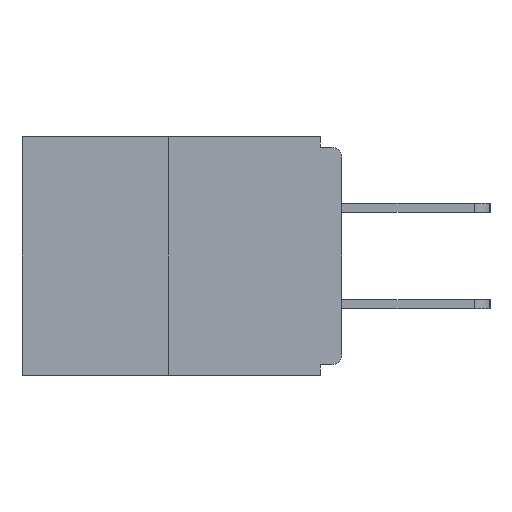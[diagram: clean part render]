
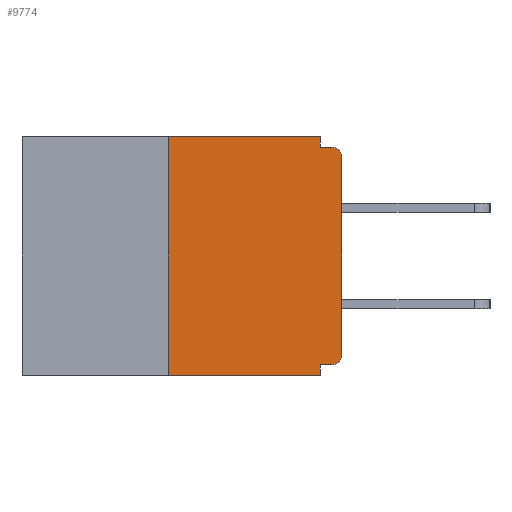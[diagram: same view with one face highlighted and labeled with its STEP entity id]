
A CAD part, left-side view. The second image highlights one B-rep face of the part: STEP entity #9774.
In plain terms, the highlighted planar face has unit normal (-1, 0, 0).
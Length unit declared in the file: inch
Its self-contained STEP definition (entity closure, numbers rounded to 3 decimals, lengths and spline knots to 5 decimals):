
#645 = ORIENTED_EDGE ( 'NONE', *, *, #3847, .F. ) ;
#1141 = VECTOR ( 'NONE', #11900, 39.37008 ) ;
#1567 = EDGE_CURVE ( 'NONE', #14206, #4129, #3228, .T. ) ;
#2393 = LINE ( 'NONE', #6548, #3280 ) ;
#2454 = DIRECTION ( 'NONE',  ( 0., -1., 0. ) ) ;
#2554 = AXIS2_PLACEMENT_3D ( 'NONE', #10308, #8791, #17284 ) ;
#2558 = DIRECTION ( 'NONE',  ( 0., 0., 1. ) ) ;
#2584 = VERTEX_POINT ( 'NONE', #14628 ) ;
#2703 = VERTEX_POINT ( 'NONE', #7894 ) ;
#2985 = CARTESIAN_POINT ( 'NONE',  ( 0., 0.031, -0.328 ) ) ;
#3004 = DIRECTION ( 'NONE',  ( -1., 0., 0. ) ) ;
#3228 = CIRCLE ( 'NONE', #16253, 0.015 ) ;
#3280 = VECTOR ( 'NONE', #12110, 39.37008 ) ;
#3322 = PLANE ( 'NONE',  #2554 ) ;
#3410 = EDGE_CURVE ( 'NONE', #3979, #9281, #3628, .T. ) ;
#3470 = VECTOR ( 'NONE', #2454, 39.37008 ) ;
#3628 = LINE ( 'NONE', #5247, #3470 ) ;
#3847 = EDGE_CURVE ( 'NONE', #2703, #13763, #7353, .T. ) ;
#3947 = VECTOR ( 'NONE', #14082, 39.37008 ) ;
#3979 = VERTEX_POINT ( 'NONE', #7965 ) ;
#4129 = VERTEX_POINT ( 'NONE', #14866 ) ;
#4178 = CARTESIAN_POINT ( 'NONE',  ( 0., 0.015, -0.313 ) ) ;
#4194 = CARTESIAN_POINT ( 'NONE',  ( 0., 0.031, -0.343 ) ) ;
#4447 = DIRECTION ( 'NONE',  ( 0., 0., -1. ) ) ;
#4765 = FACE_OUTER_BOUND ( 'NONE', #6492, .T. ) ;
#5152 = ORIENTED_EDGE ( 'NONE', *, *, #13144, .F. ) ;
#5247 = CARTESIAN_POINT ( 'NONE',  ( 0., 0.46, -0.343 ) ) ;
#5688 = VECTOR ( 'NONE', #2558, 39.37008 ) ;
#5860 = VECTOR ( 'NONE', #14161, 39.37008 ) ;
#6120 = LINE ( 'NONE', #17193, #14213 ) ;
#6492 = EDGE_LOOP ( 'NONE', ( #17473, #10334, #14534, #16892, #6606, #6872, #6657, #11064, #5152, #645 ) ) ;
#6548 = CARTESIAN_POINT ( 'NONE',  ( 0., 0.46, 0. ) ) ;
#6606 = ORIENTED_EDGE ( 'NONE', *, *, #14551, .F. ) ;
#6657 = ORIENTED_EDGE ( 'NONE', *, *, #17885, .T. ) ;
#6781 = EDGE_CURVE ( 'NONE', #9691, #9281, #13333, .T. ) ;
#6872 = ORIENTED_EDGE ( 'NONE', *, *, #1567, .T. ) ;
#6930 = AXIS2_PLACEMENT_3D ( 'NONE', #12238, #14766, #17742 ) ;
#7265 = CARTESIAN_POINT ( 'NONE',  ( 0., 0., -0.328 ) ) ;
#7353 = LINE ( 'NONE', #8737, #3947 ) ;
#7894 = CARTESIAN_POINT ( 'NONE',  ( 0., 0.031, 0. ) ) ;
#7965 = CARTESIAN_POINT ( 'NONE',  ( 0., 0.25, -0.343 ) ) ;
#8478 = VERTEX_POINT ( 'NONE', #16604 ) ;
#8737 = CARTESIAN_POINT ( 'NONE',  ( 0., 0.031, 0. ) ) ;
#8791 = DIRECTION ( 'NONE',  ( 1., 0., 0. ) ) ;
#9272 = EDGE_CURVE ( 'NONE', #3979, #2584, #14990, .T. ) ;
#9281 = VERTEX_POINT ( 'NONE', #4194 ) ;
#9298 = VECTOR ( 'NONE', #4447, 39.37008 ) ;
#9691 = VERTEX_POINT ( 'NONE', #2985 ) ;
#9716 = DIRECTION ( 'NONE',  ( 0., 0., -1. ) ) ;
#9774 = ADVANCED_FACE ( 'NONE', ( #4765 ), #3322, .F. ) ;
#10272 = CARTESIAN_POINT ( 'NONE',  ( 0., 0.015, -0.328 ) ) ;
#10308 = CARTESIAN_POINT ( 'NONE',  ( 0., 0.46, 0. ) ) ;
#10334 = ORIENTED_EDGE ( 'NONE', *, *, #9272, .F. ) ;
#11064 = ORIENTED_EDGE ( 'NONE', *, *, #17128, .T. ) ;
#11674 = CARTESIAN_POINT ( 'NONE',  ( 0., 0.031, -0.015 ) ) ;
#11900 = DIRECTION ( 'NONE',  ( 0., 0., 1. ) ) ;
#12110 = DIRECTION ( 'NONE',  ( 0., -1., 0. ) ) ;
#12238 = CARTESIAN_POINT ( 'NONE',  ( 0., 0.015, -0.03 ) ) ;
#12731 = VERTEX_POINT ( 'NONE', #16027 ) ;
#13144 = EDGE_CURVE ( 'NONE', #13763, #12731, #6120, .T. ) ;
#13333 = LINE ( 'NONE', #14588, #9298 ) ;
#13763 = VERTEX_POINT ( 'NONE', #11674 ) ;
#14082 = DIRECTION ( 'NONE',  ( 0., 0., -1. ) ) ;
#14161 = DIRECTION ( 'NONE',  ( 0., 1., 0. ) ) ;
#14179 = CIRCLE ( 'NONE', #6930, 0.015 ) ;
#14206 = VERTEX_POINT ( 'NONE', #10272 ) ;
#14213 = VECTOR ( 'NONE', #15926, 39.37008 ) ;
#14534 = ORIENTED_EDGE ( 'NONE', *, *, #3410, .T. ) ;
#14551 = EDGE_CURVE ( 'NONE', #14206, #9691, #15867, .T. ) ;
#14588 = CARTESIAN_POINT ( 'NONE',  ( 0., 0.031, -0.343 ) ) ;
#14628 = CARTESIAN_POINT ( 'NONE',  ( 0., 0.25, 0. ) ) ;
#14766 = DIRECTION ( 'NONE',  ( -1., 0., 0. ) ) ;
#14866 = CARTESIAN_POINT ( 'NONE',  ( 0., 0., -0.313 ) ) ;
#14990 = LINE ( 'NONE', #16539, #5688 ) ;
#15059 = EDGE_CURVE ( 'NONE', #2584, #2703, #2393, .T. ) ;
#15867 = LINE ( 'NONE', #7265, #5860 ) ;
#15926 = DIRECTION ( 'NONE',  ( 0., -1., 0. ) ) ;
#15960 = CARTESIAN_POINT ( 'NONE',  ( 0., 0., 0. ) ) ;
#16027 = CARTESIAN_POINT ( 'NONE',  ( 0., 0.015, -0.015 ) ) ;
#16253 = AXIS2_PLACEMENT_3D ( 'NONE', #4178, #3004, #9716 ) ;
#16539 = CARTESIAN_POINT ( 'NONE',  ( 0., 0.25, 0. ) ) ;
#16604 = CARTESIAN_POINT ( 'NONE',  ( 0., 0., -0.03 ) ) ;
#16892 = ORIENTED_EDGE ( 'NONE', *, *, #6781, .F. ) ;
#17128 = EDGE_CURVE ( 'NONE', #8478, #12731, #14179, .T. ) ;
#17193 = CARTESIAN_POINT ( 'NONE',  ( 0., 0., -0.015 ) ) ;
#17284 = DIRECTION ( 'NONE',  ( 0., 0., -1. ) ) ;
#17473 = ORIENTED_EDGE ( 'NONE', *, *, #15059, .F. ) ;
#17667 = LINE ( 'NONE', #15960, #1141 ) ;
#17742 = DIRECTION ( 'NONE',  ( 0., 0., -1. ) ) ;
#17885 = EDGE_CURVE ( 'NONE', #4129, #8478, #17667, .T. ) ;
